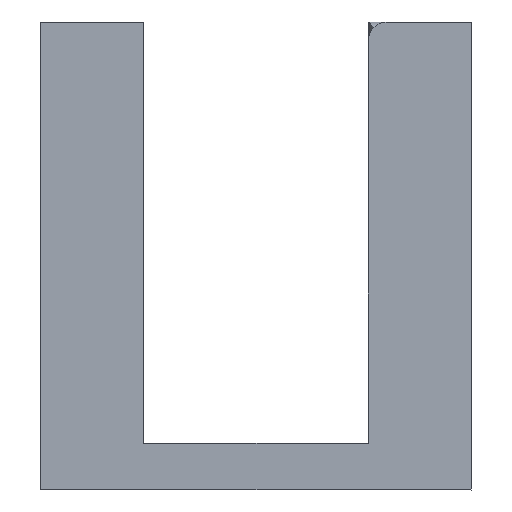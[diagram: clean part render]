
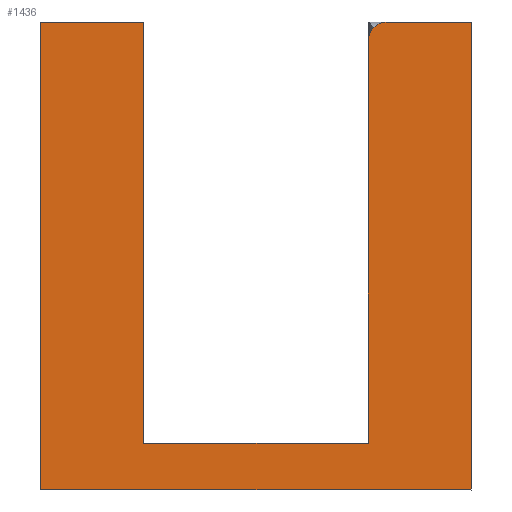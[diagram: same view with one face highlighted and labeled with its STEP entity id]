
A CAD part, left-side view. The second image highlights one B-rep face of the part: STEP entity #1436.
In plain terms, the highlighted planar face has unit normal (-1, 0, 0).
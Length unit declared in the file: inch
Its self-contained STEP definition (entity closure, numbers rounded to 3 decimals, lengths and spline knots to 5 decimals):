
#12 = EDGE_CURVE ( 'NONE', #81, #1959, #432, .T. ) ;
#60 = CARTESIAN_POINT ( 'NONE',  ( -0.62992, -0.19733, -0.03889 ) ) ;
#81 = VERTEX_POINT ( 'NONE', #451 ) ;
#105 = CARTESIAN_POINT ( 'NONE',  ( -0.62992, 0.0192, 0.05954 ) ) ;
#116 = CARTESIAN_POINT ( 'NONE',  ( -0.62992, 0.49165, 0.9444 ) ) ;
#118 = DIRECTION ( 'NONE',  ( 0., -1., 0. ) ) ;
#139 = FACE_OUTER_BOUND ( 'NONE', #767, .T. ) ;
#212 = DIRECTION ( 'NONE',  ( -1., 0., 0. ) ) ;
#233 = VECTOR ( 'NONE', #1602, 39.37008 ) ;
#238 = DIRECTION ( 'NONE',  ( 0., 0., -1. ) ) ;
#301 = DIRECTION ( 'NONE',  ( 0., 0., -1. ) ) ;
#332 = EDGE_CURVE ( 'NONE', #1183, #2010, #1403, .T. ) ;
#392 = VERTEX_POINT ( 'NONE', #1907 ) ;
#430 = VECTOR ( 'NONE', #118, 39.37008 ) ;
#432 = LINE ( 'NONE', #116, #726 ) ;
#451 = CARTESIAN_POINT ( 'NONE',  ( -0.62992, 0.49165, 0.9444 ) ) ;
#484 = VECTOR ( 'NONE', #2215, 39.37008 ) ;
#556 = CARTESIAN_POINT ( 'NONE',  ( -0.62992, 0.70818, 0.9444 ) ) ;
#598 = DIRECTION ( 'NONE',  ( -1., 0., 0. ) ) ;
#599 = ORIENTED_EDGE ( 'NONE', *, *, #1068, .F. ) ;
#642 = DIRECTION ( 'NONE',  ( 0., 1., 0. ) ) ;
#647 = ORIENTED_EDGE ( 'NONE', *, *, #1037, .F. ) ;
#665 = CARTESIAN_POINT ( 'NONE',  ( -0.62992, 0.70818, -0.03889 ) ) ;
#726 = VECTOR ( 'NONE', #238, 39.37008 ) ;
#767 = EDGE_LOOP ( 'NONE', ( #1642, #2176, #1675, #647, #2011, #2195, #599, #818, #1864 ) ) ;
#797 = LINE ( 'NONE', #60, #233 ) ;
#801 = EDGE_CURVE ( 'NONE', #1542, #2010, #797, .T. ) ;
#818 = ORIENTED_EDGE ( 'NONE', *, *, #2075, .F. ) ;
#821 = CARTESIAN_POINT ( 'NONE',  ( -0.62992, 0.0192, 0.05954 ) ) ;
#830 = VECTOR ( 'NONE', #301, 39.37008 ) ;
#842 = CARTESIAN_POINT ( 'NONE',  ( -0.62992, -0.02017, 0.9444 ) ) ;
#878 = EDGE_CURVE ( 'NONE', #1142, #392, #2201, .T. ) ;
#935 = CARTESIAN_POINT ( 'NONE',  ( -0.62992, -0.19733, -0.03889 ) ) ;
#940 = LINE ( 'NONE', #1319, #430 ) ;
#973 = VECTOR ( 'NONE', #1897, 39.37008 ) ;
#991 = LINE ( 'NONE', #821, #1344 ) ;
#1006 = VERTEX_POINT ( 'NONE', #105 ) ;
#1020 = CARTESIAN_POINT ( 'NONE',  ( -0.62992, 0.70818, 0.9444 ) ) ;
#1032 = CARTESIAN_POINT ( 'NONE',  ( -0.62992, 0.70818, 0.9444 ) ) ;
#1037 = EDGE_CURVE ( 'NONE', #1183, #81, #940, .T. ) ;
#1043 = AXIS2_PLACEMENT_3D ( 'NONE', #1627, #598, #1801 ) ;
#1068 = EDGE_CURVE ( 'NONE', #2043, #1542, #1744, .T. ) ;
#1081 = EDGE_CURVE ( 'NONE', #1006, #1959, #991, .T. ) ;
#1142 = VERTEX_POINT ( 'NONE', #842 ) ;
#1183 = VERTEX_POINT ( 'NONE', #1020 ) ;
#1243 = PLANE ( 'NONE',  #2095 ) ;
#1319 = CARTESIAN_POINT ( 'NONE',  ( -0.62992, 0.70818, 0.9444 ) ) ;
#1344 = VECTOR ( 'NONE', #642, 39.37008 ) ;
#1399 = CARTESIAN_POINT ( 'NONE',  ( -0.62992, 0.49165, 0.05954 ) ) ;
#1403 = LINE ( 'NONE', #1032, #484 ) ;
#1421 = DIRECTION ( 'NONE',  ( 0., 0., -1. ) ) ;
#1436 = ADVANCED_FACE ( 'NONE', ( #139 ), #1243, .T. ) ;
#1526 = CARTESIAN_POINT ( 'NONE',  ( -0.62992, -0.19733, 0.9444 ) ) ;
#1534 = CARTESIAN_POINT ( 'NONE',  ( -0.62992, -0.02017, 0.9444 ) ) ;
#1542 = VERTEX_POINT ( 'NONE', #935 ) ;
#1602 = DIRECTION ( 'NONE',  ( 0., 1., 0. ) ) ;
#1627 = CARTESIAN_POINT ( 'NONE',  ( -0.62992, -0.02017, 0.90503 ) ) ;
#1642 = ORIENTED_EDGE ( 'NONE', *, *, #1944, .T. ) ;
#1644 = VECTOR ( 'NONE', #2069, 39.37008 ) ;
#1675 = ORIENTED_EDGE ( 'NONE', *, *, #12, .F. ) ;
#1744 = LINE ( 'NONE', #2006, #830 ) ;
#1801 = DIRECTION ( 'NONE',  ( 0., 0., 1. ) ) ;
#1864 = ORIENTED_EDGE ( 'NONE', *, *, #878, .T. ) ;
#1890 = LINE ( 'NONE', #1534, #973 ) ;
#1897 = DIRECTION ( 'NONE',  ( 0., -1., 0. ) ) ;
#1907 = CARTESIAN_POINT ( 'NONE',  ( -0.62992, 0.0192, 0.90503 ) ) ;
#1910 = CARTESIAN_POINT ( 'NONE',  ( -0.62992, 0.0192, 0.90503 ) ) ;
#1922 = LINE ( 'NONE', #1910, #1644 ) ;
#1944 = EDGE_CURVE ( 'NONE', #392, #1006, #1922, .T. ) ;
#1959 = VERTEX_POINT ( 'NONE', #1399 ) ;
#2006 = CARTESIAN_POINT ( 'NONE',  ( -0.62992, -0.19733, 0.9444 ) ) ;
#2010 = VERTEX_POINT ( 'NONE', #665 ) ;
#2011 = ORIENTED_EDGE ( 'NONE', *, *, #332, .T. ) ;
#2043 = VERTEX_POINT ( 'NONE', #1526 ) ;
#2069 = DIRECTION ( 'NONE',  ( 0., 0., -1. ) ) ;
#2075 = EDGE_CURVE ( 'NONE', #1142, #2043, #1890, .T. ) ;
#2095 = AXIS2_PLACEMENT_3D ( 'NONE', #556, #212, #1421 ) ;
#2176 = ORIENTED_EDGE ( 'NONE', *, *, #1081, .T. ) ;
#2195 = ORIENTED_EDGE ( 'NONE', *, *, #801, .F. ) ;
#2201 = CIRCLE ( 'NONE', #1043, 0.03937 ) ;
#2215 = DIRECTION ( 'NONE',  ( 0., 0., -1. ) ) ;
